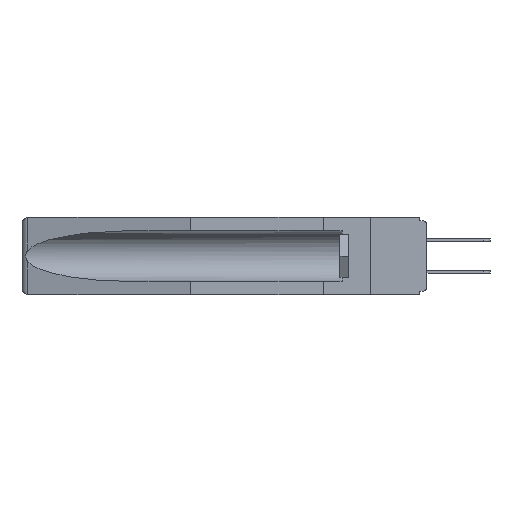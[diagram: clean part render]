
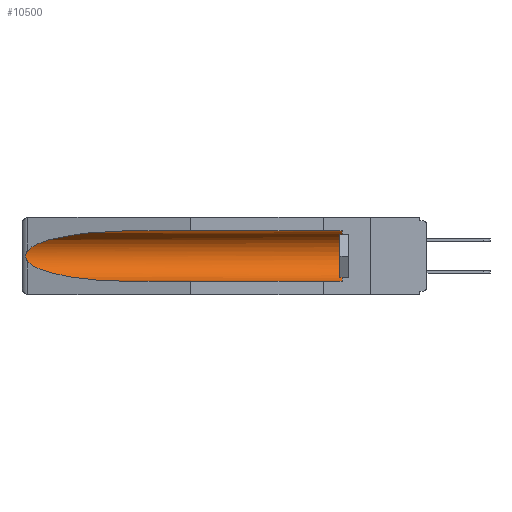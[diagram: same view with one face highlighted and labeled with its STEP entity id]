
A CAD part, left-side view. The second image highlights one B-rep face of the part: STEP entity #10500.
In plain terms, the highlighted cylindrical face has radius 2.857 mm (diameter 5.715 mm), a partial arc.
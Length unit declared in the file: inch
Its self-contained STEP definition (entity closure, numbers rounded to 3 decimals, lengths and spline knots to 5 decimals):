
#1013 = LINE ( 'NONE', #2353, #21092 ) ;
#1386 = EDGE_CURVE ( 'NONE', #23296, #10496, #6685, .T. ) ;
#1691 = DIRECTION ( 'NONE',  ( 0., 1., 0. ) ) ;
#1756 = CARTESIAN_POINT ( 'NONE',  ( 0.26537, 1.52718, -0.19328 ) ) ;
#1780 = AXIS2_PLACEMENT_3D ( 'NONE', #11973, #1691, #10379 ) ;
#2291 = LINE ( 'NONE', #6397, #11302 ) ;
#2353 = CARTESIAN_POINT ( 'NONE',  ( 0.155, -0.30754, -0.059 ) ) ;
#2776 = VERTEX_POINT ( 'NONE', #22731 ) ;
#2985 =( BOUNDED_CURVE ( )  B_SPLINE_CURVE ( 3, ( #25915, #17752, #9549, #5048 ),
 .UNSPECIFIED., .F., .F. ) 
 B_SPLINE_CURVE_WITH_KNOTS ( ( 4, 4 ),
 ( 4.71239, 6.08839 ),
 .UNSPECIFIED. ) 
 CURVE ( )  GEOMETRIC_REPRESENTATION_ITEM ( )  RATIONAL_B_SPLINE_CURVE ( ( 1., 0.848, 0.848, 1. ) ) 
 REPRESENTATION_ITEM ( '' )  );
#3132 = CARTESIAN_POINT ( 'NONE',  ( 0.155, 0.126, -0.284 ) ) ;
#3260 = CARTESIAN_POINT ( 'NONE',  ( 0.155, 1.07973, -0.059 ) ) ;
#3323 = CARTESIAN_POINT ( 'NONE',  ( 0.2675, 1.53308, -0.16763 ) ) ;
#3440 = EDGE_CURVE ( 'NONE', #3846, #2776, #2985, .T. ) ;
#3846 = VERTEX_POINT ( 'NONE', #3260 ) ;
#4020 = CARTESIAN_POINT ( 'NONE',  ( 0.155, 1.07973, -0.284 ) ) ;
#5048 = CARTESIAN_POINT ( 'NONE',  ( 0.26537, 1.52718, -0.14972 ) ) ;
#6352 = ORIENTED_EDGE ( 'NONE', *, *, #3440, .T. ) ;
#6397 = CARTESIAN_POINT ( 'NONE',  ( 0.155, -0.30754, -0.284 ) ) ;
#6685 =( BOUNDED_CURVE ( )  B_SPLINE_CURVE ( 3, ( #1756, #26727, #22631, #4020 ),
 .UNSPECIFIED., .F., .F. ) 
 B_SPLINE_CURVE_WITH_KNOTS ( ( 4, 4 ),
 ( 0.1948, 1.5708 ),
 .UNSPECIFIED. ) 
 CURVE ( )  GEOMETRIC_REPRESENTATION_ITEM ( )  RATIONAL_B_SPLINE_CURVE ( ( 1., 0.848, 0.848, 1. ) ) 
 REPRESENTATION_ITEM ( '' )  );
#7803 = EDGE_CURVE ( 'NONE', #16320, #10496, #2291, .T. ) ;
#9523 = VERTEX_POINT ( 'NONE', #16636 ) ;
#9549 = CARTESIAN_POINT ( 'NONE',  ( 0.25451, 1.48313, -0.09465 ) ) ;
#9750 = DIRECTION ( 'NONE',  ( 0., -1., 0. ) ) ;
#10379 = DIRECTION ( 'NONE',  ( 0., 0., 1. ) ) ;
#10482 = ORIENTED_EDGE ( 'NONE', *, *, #16148, .T. ) ;
#10496 = VERTEX_POINT ( 'NONE', #18492 ) ;
#10500 = ADVANCED_FACE ( 'NONE', ( #25470 ), #15425, .F. ) ;
#11105 = CIRCLE ( 'NONE', #14442, 0.1125 ) ;
#11284 = ORIENTED_EDGE ( 'NONE', *, *, #7803, .F. ) ;
#11302 = VECTOR ( 'NONE', #21021, 39.37008 ) ;
#11701 = CARTESIAN_POINT ( 'NONE',  ( 0.26597, 1.5296, -0.19026 ) ) ;
#11876 = CARTESIAN_POINT ( 'NONE',  ( 0.2675, 1.53308, -0.17534 ) ) ;
#11973 = CARTESIAN_POINT ( 'NONE',  ( 0.155, -0.30754, -0.1715 ) ) ;
#12059 = EDGE_CURVE ( 'NONE', #16320, #9523, #11105, .T. ) ;
#12429 = ORIENTED_EDGE ( 'NONE', *, *, #19678, .T. ) ;
#13776 = CARTESIAN_POINT ( 'NONE',  ( 0.26597, 1.52961, -0.15275 ) ) ;
#13867 = CARTESIAN_POINT ( 'NONE',  ( 0.155, 0.126, -0.1715 ) ) ;
#14009 = CARTESIAN_POINT ( 'NONE',  ( 0.26537, 1.52718, -0.19328 ) ) ;
#14442 = AXIS2_PLACEMENT_3D ( 'NONE', #13867, #9750, #22212 ) ;
#15016 = ORIENTED_EDGE ( 'NONE', *, *, #12059, .T. ) ;
#15425 = CYLINDRICAL_SURFACE ( 'NONE', #1780, 0.1125 ) ;
#15622 = CARTESIAN_POINT ( 'NONE',  ( 0.26654, 1.53092, -0.15636 ) ) ;
#15989 = CARTESIAN_POINT ( 'NONE',  ( 0.26537, 1.52718, -0.14972 ) ) ;
#16148 = EDGE_CURVE ( 'NONE', #9523, #3846, #1013, .T. ) ;
#16320 = VERTEX_POINT ( 'NONE', #3132 ) ;
#16636 = CARTESIAN_POINT ( 'NONE',  ( 0.155, 0.126, -0.059 ) ) ;
#17752 = CARTESIAN_POINT ( 'NONE',  ( 0.21114, 1.30732, -0.059 ) ) ;
#18492 = CARTESIAN_POINT ( 'NONE',  ( 0.155, 1.07973, -0.284 ) ) ;
#18704 = DIRECTION ( 'NONE',  ( 0., 1., 0. ) ) ;
#19192 = EDGE_LOOP ( 'NONE', ( #6352, #12429, #21028, #11284, #15016, #10482 ) ) ;
#19678 = EDGE_CURVE ( 'NONE', #2776, #23296, #23837, .T. ) ;
#21021 = DIRECTION ( 'NONE',  ( 0., 1., 0. ) ) ;
#21028 = ORIENTED_EDGE ( 'NONE', *, *, #1386, .T. ) ;
#21092 = VECTOR ( 'NONE', #18704, 39.37008 ) ;
#22046 = CARTESIAN_POINT ( 'NONE',  ( 0.2673, 1.5327, -0.16383 ) ) ;
#22133 = CARTESIAN_POINT ( 'NONE',  ( 0.2673, 1.53269, -0.17917 ) ) ;
#22212 = DIRECTION ( 'NONE',  ( 0., 0., 1. ) ) ;
#22631 = CARTESIAN_POINT ( 'NONE',  ( 0.21114, 1.30732, -0.284 ) ) ;
#22731 = CARTESIAN_POINT ( 'NONE',  ( 0.26537, 1.52718, -0.14972 ) ) ;
#23296 = VERTEX_POINT ( 'NONE', #14009 ) ;
#23837 = B_SPLINE_CURVE_WITH_KNOTS ( 'NONE', 3,
 ( #15989, #13776, #15622, #22046, #3323, #11876, #22133, #26026, #11701, #26225 ),
 .UNSPECIFIED., .F., .F.,
 ( 4, 2, 2, 2, 4 ),
 ( 0., 0.00029, 0.00058, 0.00087, 0.00117 ),
 .UNSPECIFIED. ) ;
#25470 = FACE_OUTER_BOUND ( 'NONE', #19192, .T. ) ;
#25915 = CARTESIAN_POINT ( 'NONE',  ( 0.155, 1.07973, -0.059 ) ) ;
#26026 = CARTESIAN_POINT ( 'NONE',  ( 0.26655, 1.53094, -0.18657 ) ) ;
#26225 = CARTESIAN_POINT ( 'NONE',  ( 0.26537, 1.52718, -0.19328 ) ) ;
#26727 = CARTESIAN_POINT ( 'NONE',  ( 0.25451, 1.48313, -0.24835 ) ) ;
